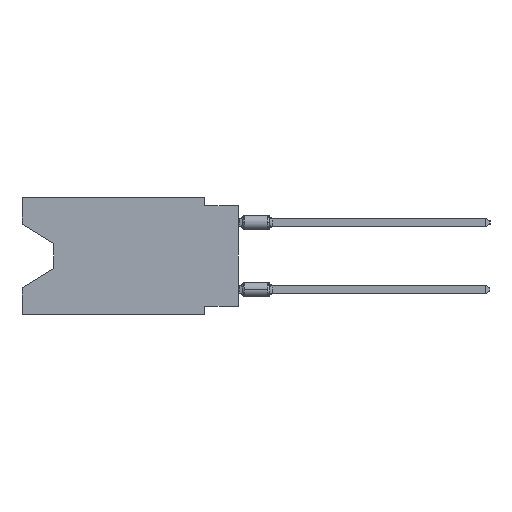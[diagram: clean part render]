
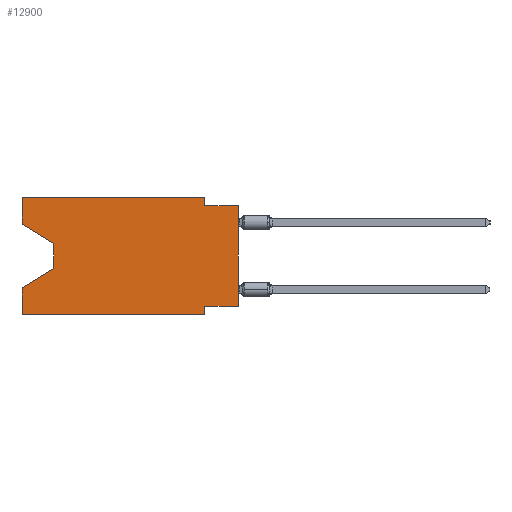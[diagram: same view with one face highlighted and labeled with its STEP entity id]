
A CAD part, left-side view. The second image highlights one B-rep face of the part: STEP entity #12900.
In plain terms, the highlighted planar face has unit normal (-1, 0, 0).
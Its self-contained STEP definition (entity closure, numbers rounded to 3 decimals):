
#180 = EDGE_CURVE ( 'NONE', #5273, #6760, #17133, .T. ) ;
#243 = EDGE_CURVE ( 'NONE', #483, #2526, #11633, .T. ) ;
#483 = VERTEX_POINT ( 'NONE', #14420 ) ;
#502 = CARTESIAN_POINT ( 'NONE',  ( 0., 16.383, -8.89 ) ) ;
#1084 = LINE ( 'NONE', #13858, #17744 ) ;
#1923 = VECTOR ( 'NONE', #22152, 1000. ) ;
#2074 = VERTEX_POINT ( 'NONE', #5314 ) ;
#2156 = CARTESIAN_POINT ( 'NONE',  ( 0., 13.97, -5.385 ) ) ;
#2383 = LINE ( 'NONE', #8042, #14627 ) ;
#2526 = VERTEX_POINT ( 'NONE', #20992 ) ;
#2973 = LINE ( 'NONE', #13900, #4879 ) ;
#3090 = DIRECTION ( 'NONE',  ( 0., -0.855, -0.519 ) ) ;
#3468 = LINE ( 'NONE', #5423, #6661 ) ;
#3897 = VERTEX_POINT ( 'NONE', #15034 ) ;
#3989 = CARTESIAN_POINT ( 'NONE',  ( 0., 13.97, -5.385 ) ) ;
#4042 = CARTESIAN_POINT ( 'NONE',  ( 0., 16.383, -2.038 ) ) ;
#4625 = VECTOR ( 'NONE', #5839, 1000. ) ;
#4683 = ORIENTED_EDGE ( 'NONE', *, *, #9494, .F. ) ;
#4879 = VECTOR ( 'NONE', #3090, 1000. ) ;
#4955 = VECTOR ( 'NONE', #15721, 1000. ) ;
#5000 = ORIENTED_EDGE ( 'NONE', *, *, #23842, .T. ) ;
#5273 = VERTEX_POINT ( 'NONE', #2156 ) ;
#5314 = CARTESIAN_POINT ( 'NONE',  ( 0., 0., -8.255 ) ) ;
#5423 = CARTESIAN_POINT ( 'NONE',  ( 0., 0., -8.255 ) ) ;
#5679 = LINE ( 'NONE', #13044, #18564 ) ;
#5773 = DIRECTION ( 'NONE',  ( 0., 0., -1. ) ) ;
#5839 = DIRECTION ( 'NONE',  ( 0., -1., 0. ) ) ;
#6127 = EDGE_CURVE ( 'NONE', #2074, #2526, #12808, .T. ) ;
#6495 = DIRECTION ( 'NONE',  ( 0., -1., 0. ) ) ;
#6661 = VECTOR ( 'NONE', #9226, 1000. ) ;
#6760 = VERTEX_POINT ( 'NONE', #7066 ) ;
#6794 = AXIS2_PLACEMENT_3D ( 'NONE', #15091, #22619, #5773 ) ;
#6913 = EDGE_CURVE ( 'NONE', #8056, #6760, #13909, .T. ) ;
#6959 = VECTOR ( 'NONE', #10113, 1000. ) ;
#7066 = CARTESIAN_POINT ( 'NONE',  ( 0., 16.383, -6.852 ) ) ;
#7410 = VECTOR ( 'NONE', #22693, 1000. ) ;
#7503 = LINE ( 'NONE', #9347, #10314 ) ;
#7614 = PLANE ( 'NONE',  #6794 ) ;
#8042 = CARTESIAN_POINT ( 'NONE',  ( 0., 16.383, -8.89 ) ) ;
#8056 = VERTEX_POINT ( 'NONE', #502 ) ;
#8210 = VERTEX_POINT ( 'NONE', #22143 ) ;
#8252 = CARTESIAN_POINT ( 'NONE',  ( 0., 2.54, -8.89 ) ) ;
#8549 = VECTOR ( 'NONE', #22694, 1000. ) ;
#9226 = DIRECTION ( 'NONE',  ( 0., 1., 0. ) ) ;
#9270 = EDGE_CURVE ( 'NONE', #12893, #8210, #22328, .T. ) ;
#9347 = CARTESIAN_POINT ( 'NONE',  ( 0., 2.54, 0. ) ) ;
#9373 = ORIENTED_EDGE ( 'NONE', *, *, #12536, .T. ) ;
#9494 = EDGE_CURVE ( 'NONE', #2074, #11551, #3468, .T. ) ;
#9863 = EDGE_LOOP ( 'NONE', ( #5000, #9373, #22274, #16809, #14228, #13835, #4683, #12180, #19906, #21193, #12573, #14792 ) ) ;
#10113 = DIRECTION ( 'NONE',  ( 0., 0., 1. ) ) ;
#10314 = VECTOR ( 'NONE', #20776, 1000. ) ;
#10609 = CARTESIAN_POINT ( 'NONE',  ( 0., 2.54, 0. ) ) ;
#11551 = VERTEX_POINT ( 'NONE', #20158 ) ;
#11633 = LINE ( 'NONE', #19101, #4625 ) ;
#12180 = ORIENTED_EDGE ( 'NONE', *, *, #6127, .T. ) ;
#12536 = EDGE_CURVE ( 'NONE', #3897, #5273, #5679, .T. ) ;
#12573 = ORIENTED_EDGE ( 'NONE', *, *, #14921, .F. ) ;
#12808 = LINE ( 'NONE', #14751, #1923 ) ;
#12893 = VERTEX_POINT ( 'NONE', #4042 ) ;
#12900 = ADVANCED_FACE ( 'NONE', ( #20511 ), #7614, .F. ) ;
#13044 = CARTESIAN_POINT ( 'NONE',  ( 0., 13.97, -3.505 ) ) ;
#13835 = ORIENTED_EDGE ( 'NONE', *, *, #21354, .F. ) ;
#13858 = CARTESIAN_POINT ( 'NONE',  ( 0., 16.383, 0. ) ) ;
#13900 = CARTESIAN_POINT ( 'NONE',  ( 0., 16.383, -2.038 ) ) ;
#13909 = LINE ( 'NONE', #21419, #6959 ) ;
#14228 = ORIENTED_EDGE ( 'NONE', *, *, #16828, .T. ) ;
#14420 = CARTESIAN_POINT ( 'NONE',  ( 0., 2.54, -0.635 ) ) ;
#14627 = VECTOR ( 'NONE', #18719, 1000. ) ;
#14751 = CARTESIAN_POINT ( 'NONE',  ( 0., 0., 0. ) ) ;
#14792 = ORIENTED_EDGE ( 'NONE', *, *, #9270, .F. ) ;
#14921 = EDGE_CURVE ( 'NONE', #8210, #20955, #1084, .T. ) ;
#15034 = CARTESIAN_POINT ( 'NONE',  ( 0., 13.97, -3.505 ) ) ;
#15091 = CARTESIAN_POINT ( 'NONE',  ( 0., 16.383, 0. ) ) ;
#15532 = VERTEX_POINT ( 'NONE', #21842 ) ;
#15721 = DIRECTION ( 'NONE',  ( 0., 0., -1. ) ) ;
#16809 = ORIENTED_EDGE ( 'NONE', *, *, #6913, .F. ) ;
#16828 = EDGE_CURVE ( 'NONE', #8056, #15532, #2383, .T. ) ;
#16999 = CARTESIAN_POINT ( 'NONE',  ( 0., 16.383, 0. ) ) ;
#17133 = LINE ( 'NONE', #3989, #8549 ) ;
#17744 = VECTOR ( 'NONE', #6495, 1000. ) ;
#18564 = VECTOR ( 'NONE', #18693, 1000. ) ;
#18693 = DIRECTION ( 'NONE',  ( 0., 0., -1. ) ) ;
#18719 = DIRECTION ( 'NONE',  ( 0., -1., 0. ) ) ;
#19101 = CARTESIAN_POINT ( 'NONE',  ( 0., 0., -0.635 ) ) ;
#19291 = LINE ( 'NONE', #8252, #4955 ) ;
#19906 = ORIENTED_EDGE ( 'NONE', *, *, #243, .F. ) ;
#20158 = CARTESIAN_POINT ( 'NONE',  ( 0., 2.54, -8.255 ) ) ;
#20511 = FACE_OUTER_BOUND ( 'NONE', #9863, .T. ) ;
#20776 = DIRECTION ( 'NONE',  ( 0., 0., -1. ) ) ;
#20955 = VERTEX_POINT ( 'NONE', #10609 ) ;
#20992 = CARTESIAN_POINT ( 'NONE',  ( 0., 0., -0.635 ) ) ;
#21193 = ORIENTED_EDGE ( 'NONE', *, *, #22172, .F. ) ;
#21354 = EDGE_CURVE ( 'NONE', #11551, #15532, #19291, .T. ) ;
#21419 = CARTESIAN_POINT ( 'NONE',  ( 0., 16.383, 0. ) ) ;
#21842 = CARTESIAN_POINT ( 'NONE',  ( 0., 2.54, -8.89 ) ) ;
#22143 = CARTESIAN_POINT ( 'NONE',  ( 0., 16.383, 0. ) ) ;
#22152 = DIRECTION ( 'NONE',  ( 0., 0., 1. ) ) ;
#22172 = EDGE_CURVE ( 'NONE', #20955, #483, #7503, .T. ) ;
#22274 = ORIENTED_EDGE ( 'NONE', *, *, #180, .T. ) ;
#22328 = LINE ( 'NONE', #16999, #7410 ) ;
#22619 = DIRECTION ( 'NONE',  ( 1., 0., 0. ) ) ;
#22693 = DIRECTION ( 'NONE',  ( 0., 0., 1. ) ) ;
#22694 = DIRECTION ( 'NONE',  ( 0., 0.855, -0.519 ) ) ;
#23842 = EDGE_CURVE ( 'NONE', #12893, #3897, #2973, .T. ) ;
